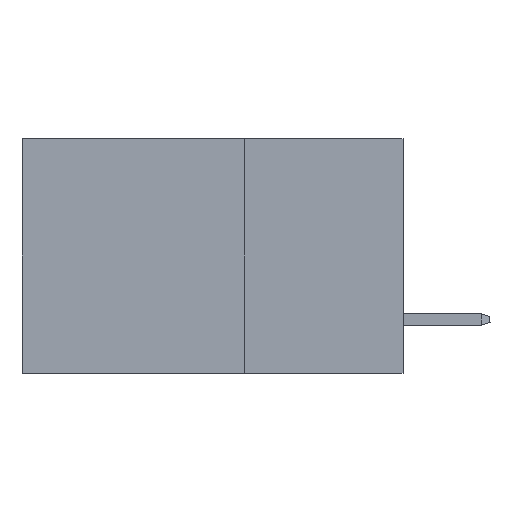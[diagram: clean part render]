
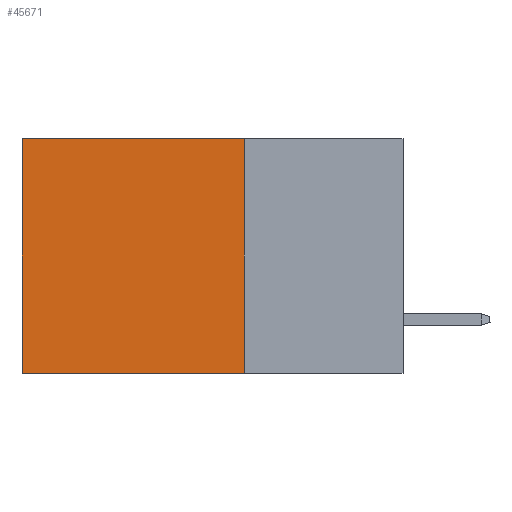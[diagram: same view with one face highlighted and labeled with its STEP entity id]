
A CAD part, left-side view. The second image highlights one B-rep face of the part: STEP entity #45671.
In plain terms, the highlighted planar face has unit normal (-1, 0, 0).
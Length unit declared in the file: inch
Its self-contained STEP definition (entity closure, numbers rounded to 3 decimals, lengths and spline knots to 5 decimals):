
#3682 = EDGE_CURVE ( 'NONE', #29811, #8707, #6415, .T. ) ;
#4634 = CARTESIAN_POINT ( 'NONE',  ( 0.2875, 0.25, -0.37 ) ) ;
#5592 = VECTOR ( 'NONE', #9225, 39.37008 ) ;
#5763 = CARTESIAN_POINT ( 'NONE',  ( 0.2875, 0.6, 0. ) ) ;
#5902 = FACE_OUTER_BOUND ( 'NONE', #38482, .T. ) ;
#5998 = VERTEX_POINT ( 'NONE', #8296 ) ;
#6200 = AXIS2_PLACEMENT_3D ( 'NONE', #23958, #31145, #34434 ) ;
#6415 = LINE ( 'NONE', #45583, #29231 ) ;
#6593 = PLANE ( 'NONE',  #6200 ) ;
#8296 = CARTESIAN_POINT ( 'NONE',  ( 0.2875, 0.25, -0.37 ) ) ;
#8707 = VERTEX_POINT ( 'NONE', #32101 ) ;
#9225 = DIRECTION ( 'NONE',  ( 0., 1., 0. ) ) ;
#12018 = EDGE_CURVE ( 'NONE', #5998, #8707, #29218, .T. ) ;
#17005 = ORIENTED_EDGE ( 'NONE', *, *, #12018, .F. ) ;
#18091 = LINE ( 'NONE', #32492, #42304 ) ;
#19343 = ORIENTED_EDGE ( 'NONE', *, *, #42973, .T. ) ;
#21107 = ORIENTED_EDGE ( 'NONE', *, *, #35865, .F. ) ;
#22289 = VECTOR ( 'NONE', #36447, 39.37008 ) ;
#23958 = CARTESIAN_POINT ( 'NONE',  ( 0.2875, 0.25, 0. ) ) ;
#26825 = LINE ( 'NONE', #41020, #5592 ) ;
#27454 = ORIENTED_EDGE ( 'NONE', *, *, #3682, .T. ) ;
#29218 = LINE ( 'NONE', #4634, #22289 ) ;
#29231 = VECTOR ( 'NONE', #38429, 39.37008 ) ;
#29811 = VERTEX_POINT ( 'NONE', #5763 ) ;
#31145 = DIRECTION ( 'NONE',  ( 1., 0., 0. ) ) ;
#32101 = CARTESIAN_POINT ( 'NONE',  ( 0.2875, 0.6, -0.37 ) ) ;
#32492 = CARTESIAN_POINT ( 'NONE',  ( 0.2875, 0.25, 0. ) ) ;
#34115 = VERTEX_POINT ( 'NONE', #34165 ) ;
#34165 = CARTESIAN_POINT ( 'NONE',  ( 0.2875, 0.25, 0. ) ) ;
#34434 = DIRECTION ( 'NONE',  ( 0., 0., -1. ) ) ;
#35511 = DIRECTION ( 'NONE',  ( 0., 0., -1. ) ) ;
#35865 = EDGE_CURVE ( 'NONE', #34115, #5998, #18091, .T. ) ;
#36447 = DIRECTION ( 'NONE',  ( 0., 1., 0. ) ) ;
#38429 = DIRECTION ( 'NONE',  ( 0., 0., -1. ) ) ;
#38482 = EDGE_LOOP ( 'NONE', ( #27454, #17005, #21107, #19343 ) ) ;
#41020 = CARTESIAN_POINT ( 'NONE',  ( 0.2875, 0.25, 0. ) ) ;
#42304 = VECTOR ( 'NONE', #35511, 39.37008 ) ;
#42973 = EDGE_CURVE ( 'NONE', #34115, #29811, #26825, .T. ) ;
#45583 = CARTESIAN_POINT ( 'NONE',  ( 0.2875, 0.6, 0. ) ) ;
#45671 = ADVANCED_FACE ( 'NONE', ( #5902 ), #6593, .F. ) ;
